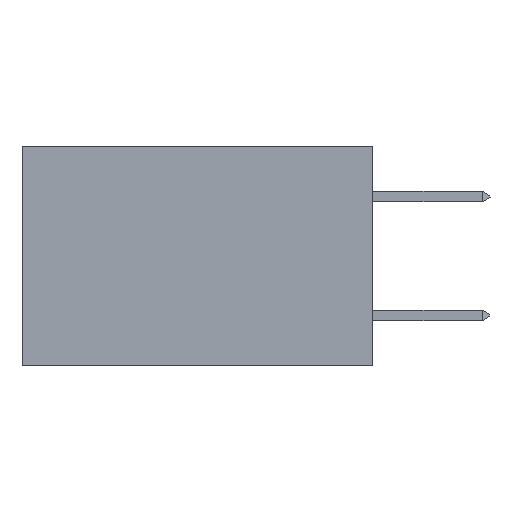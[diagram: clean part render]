
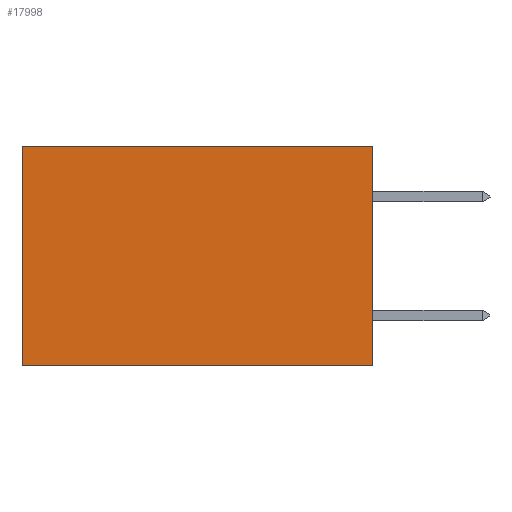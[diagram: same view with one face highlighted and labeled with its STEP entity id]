
A CAD part, left-side view. The second image highlights one B-rep face of the part: STEP entity #17998.
In plain terms, the highlighted planar face has unit normal (-1, 0, 0).
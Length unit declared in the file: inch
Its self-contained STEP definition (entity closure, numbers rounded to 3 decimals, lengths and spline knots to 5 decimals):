
#133 = CARTESIAN_POINT ( 'NONE',  ( 0.277, 0.59, -0.37 ) ) ;
#221 = VERTEX_POINT ( 'NONE', #9540 ) ;
#864 = EDGE_CURVE ( 'NONE', #221, #12530, #9981, .T. ) ;
#1324 = PLANE ( 'NONE',  #9572 ) ;
#1368 = EDGE_CURVE ( 'NONE', #10079, #221, #14440, .T. ) ;
#1615 = CARTESIAN_POINT ( 'NONE',  ( 0.277, 0., -0.37 ) ) ;
#2480 = CARTESIAN_POINT ( 'NONE',  ( 0.277, 0., -0.37 ) ) ;
#2791 = CARTESIAN_POINT ( 'NONE',  ( 0.277, 0., -0.37 ) ) ;
#4421 = ORIENTED_EDGE ( 'NONE', *, *, #12418, .F. ) ;
#4645 = EDGE_LOOP ( 'NONE', ( #10154, #11044, #4421, #8165 ) ) ;
#5533 = LINE ( 'NONE', #18463, #8813 ) ;
#5760 = DIRECTION ( 'NONE',  ( 1., 0., 0. ) ) ;
#5800 = VECTOR ( 'NONE', #16353, 39.37008 ) ;
#5807 = CARTESIAN_POINT ( 'NONE',  ( 0.277, 0., 0. ) ) ;
#6306 = VERTEX_POINT ( 'NONE', #2480 ) ;
#7315 = VECTOR ( 'NONE', #17377, 39.37008 ) ;
#7719 = CARTESIAN_POINT ( 'NONE',  ( 0.277, 0., 0. ) ) ;
#8165 = ORIENTED_EDGE ( 'NONE', *, *, #1368, .T. ) ;
#8521 = VECTOR ( 'NONE', #11657, 39.37008 ) ;
#8813 = VECTOR ( 'NONE', #12798, 39.37008 ) ;
#9540 = CARTESIAN_POINT ( 'NONE',  ( 0.277, 0.59, 0. ) ) ;
#9572 = AXIS2_PLACEMENT_3D ( 'NONE', #2791, #5760, #15661 ) ;
#9981 = LINE ( 'NONE', #16548, #5800 ) ;
#10079 = VERTEX_POINT ( 'NONE', #7719 ) ;
#10154 = ORIENTED_EDGE ( 'NONE', *, *, #864, .T. ) ;
#11044 = ORIENTED_EDGE ( 'NONE', *, *, #16657, .F. ) ;
#11657 = DIRECTION ( 'NONE',  ( 0., 1., 0. ) ) ;
#12418 = EDGE_CURVE ( 'NONE', #10079, #6306, #5533, .T. ) ;
#12530 = VERTEX_POINT ( 'NONE', #133 ) ;
#12675 = FACE_OUTER_BOUND ( 'NONE', #4645, .T. ) ;
#12798 = DIRECTION ( 'NONE',  ( 0., 0., -1. ) ) ;
#14440 = LINE ( 'NONE', #5807, #7315 ) ;
#15661 = DIRECTION ( 'NONE',  ( 0., 0., -1. ) ) ;
#16053 = LINE ( 'NONE', #1615, #8521 ) ;
#16353 = DIRECTION ( 'NONE',  ( 0., 0., -1. ) ) ;
#16548 = CARTESIAN_POINT ( 'NONE',  ( 0.277, 0.59, -0.37 ) ) ;
#16657 = EDGE_CURVE ( 'NONE', #6306, #12530, #16053, .T. ) ;
#17377 = DIRECTION ( 'NONE',  ( 0., 1., 0. ) ) ;
#17998 = ADVANCED_FACE ( 'NONE', ( #12675 ), #1324, .F. ) ;
#18463 = CARTESIAN_POINT ( 'NONE',  ( 0.277, 0., -0.37 ) ) ;
